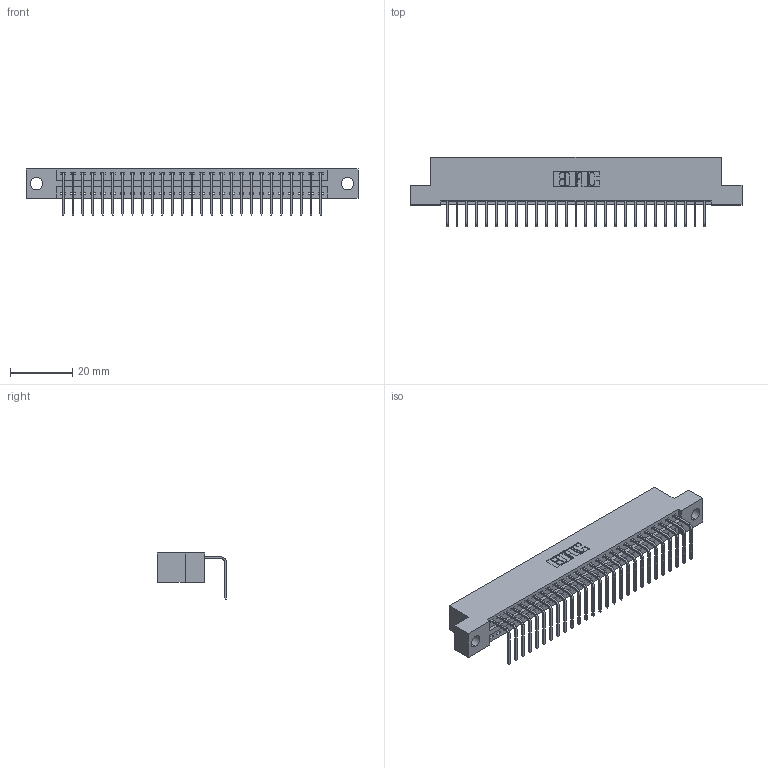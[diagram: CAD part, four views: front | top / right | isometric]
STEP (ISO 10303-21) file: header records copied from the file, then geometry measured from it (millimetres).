
FILE_DESCRIPTION (( 'STEP AP203' ), '1' );
FILE_NAME ('346-027-558-104.STEP', '2018-08-22T00:24:22', ( '' ), ( '' ), 'SwSTEP 2.0', 'SolidWorks 2016', '' );
FILE_SCHEMA (( 'CONFIG_CONTROL_DESIGN' ));
Length unit declared in the file: inch
Products named in the file (3): 346 Part_Flush Mounting Lugs - 0.156 Dia-TH; 345-292-001_558 Tail - 2; 346-027-558-104
Assembly tree (28 placements, depth 2):
  346-027-558-104
    346 Part_Flush Mounting Lugs - 0.156 Dia-TH
    345-292-001_558 Tail - 2  x27
Bounding box: 106.3 x 22.16 x 14.73 mm (x, y, z)
Volume: 10073.9 mm3; surface area: 12770.9 mm2
Topology: 28 solids, 28 shells, 1742 faces, 5243 edges, 3458 vertices
Faces by surface type: plane 1210, cylinder 532
Entity records: 18863 total; most frequent: CARTESIAN_POINT 3245, ORIENTED_EDGE 3206, DIRECTION 2881, EDGE_CURVE 1603, VECTOR 1363, LINE 1363, VERTEX_POINT 1066, AXIS2_PLACEMENT_3D 759
